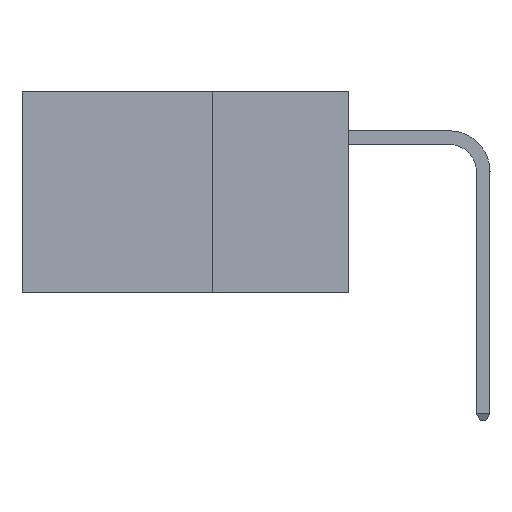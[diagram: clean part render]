
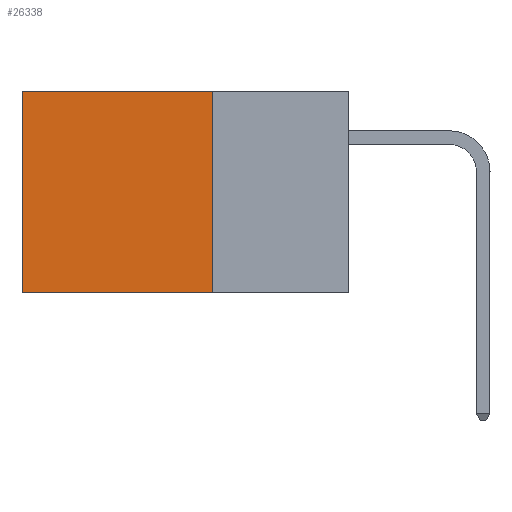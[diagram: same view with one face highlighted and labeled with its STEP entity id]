
A CAD part, left-side view. The second image highlights one B-rep face of the part: STEP entity #26338.
In plain terms, the highlighted planar face has unit normal (-1, 0, 0).
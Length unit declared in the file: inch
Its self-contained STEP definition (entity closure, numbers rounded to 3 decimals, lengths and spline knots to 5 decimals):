
#1694 = CARTESIAN_POINT ( 'NONE',  ( 0.2875, 0.25, 0. ) ) ;
#2530 = LINE ( 'NONE', #3752, #46198 ) ;
#3752 = CARTESIAN_POINT ( 'NONE',  ( 0.2875, 0.25, 0. ) ) ;
#4538 = VERTEX_POINT ( 'NONE', #1694 ) ;
#7536 = LINE ( 'NONE', #17261, #9337 ) ;
#9212 = CARTESIAN_POINT ( 'NONE',  ( 0.2875, 0.6, 0. ) ) ;
#9337 = VECTOR ( 'NONE', #24983, 39.37008 ) ;
#10099 = EDGE_LOOP ( 'NONE', ( #25663, #26197, #13103, #21746 ) ) ;
#13103 = ORIENTED_EDGE ( 'NONE', *, *, #27775, .F. ) ;
#13459 = DIRECTION ( 'NONE',  ( 1., 0., 0. ) ) ;
#17261 = CARTESIAN_POINT ( 'NONE',  ( 0.2875, 0.6, 0. ) ) ;
#18808 = EDGE_CURVE ( 'NONE', #4538, #23794, #28333, .T. ) ;
#18837 = DIRECTION ( 'NONE',  ( 0., 1., 0. ) ) ;
#21539 = LINE ( 'NONE', #30555, #45449 ) ;
#21746 = ORIENTED_EDGE ( 'NONE', *, *, #18808, .T. ) ;
#23188 = AXIS2_PLACEMENT_3D ( 'NONE', #32706, #13459, #28536 ) ;
#23794 = VERTEX_POINT ( 'NONE', #9212 ) ;
#24983 = DIRECTION ( 'NONE',  ( 0., 0., -1. ) ) ;
#25553 = VERTEX_POINT ( 'NONE', #31018 ) ;
#25663 = ORIENTED_EDGE ( 'NONE', *, *, #45455, .T. ) ;
#26197 = ORIENTED_EDGE ( 'NONE', *, *, #34590, .F. ) ;
#26338 = ADVANCED_FACE ( 'NONE', ( #32113 ), #36396, .F. ) ;
#27775 = EDGE_CURVE ( 'NONE', #4538, #42964, #2530, .T. ) ;
#28333 = LINE ( 'NONE', #32221, #44431 ) ;
#28536 = DIRECTION ( 'NONE',  ( 0., 0., -1. ) ) ;
#30555 = CARTESIAN_POINT ( 'NONE',  ( 0.2875, 0.25, -0.37 ) ) ;
#30916 = DIRECTION ( 'NONE',  ( 0., 0., -1. ) ) ;
#31018 = CARTESIAN_POINT ( 'NONE',  ( 0.2875, 0.6, -0.37 ) ) ;
#32113 = FACE_OUTER_BOUND ( 'NONE', #10099, .T. ) ;
#32221 = CARTESIAN_POINT ( 'NONE',  ( 0.2875, 0.25, 0. ) ) ;
#32706 = CARTESIAN_POINT ( 'NONE',  ( 0.2875, 0.25, 0. ) ) ;
#34590 = EDGE_CURVE ( 'NONE', #42964, #25553, #21539, .T. ) ;
#35901 = DIRECTION ( 'NONE',  ( 0., 1., 0. ) ) ;
#36396 = PLANE ( 'NONE',  #23188 ) ;
#42964 = VERTEX_POINT ( 'NONE', #47195 ) ;
#44431 = VECTOR ( 'NONE', #35901, 39.37008 ) ;
#45449 = VECTOR ( 'NONE', #18837, 39.37008 ) ;
#45455 = EDGE_CURVE ( 'NONE', #23794, #25553, #7536, .T. ) ;
#46198 = VECTOR ( 'NONE', #30916, 39.37008 ) ;
#47195 = CARTESIAN_POINT ( 'NONE',  ( 0.2875, 0.25, -0.37 ) ) ;
